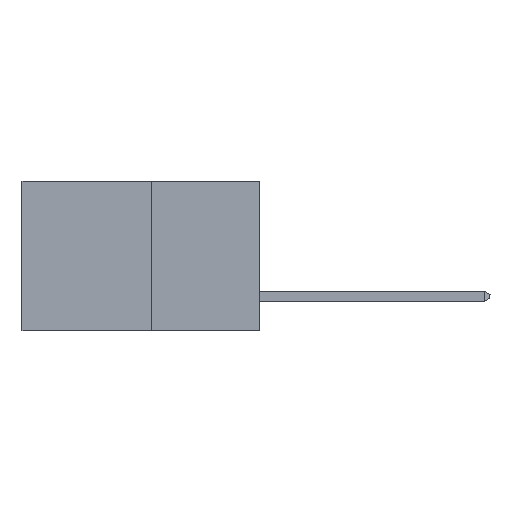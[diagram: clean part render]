
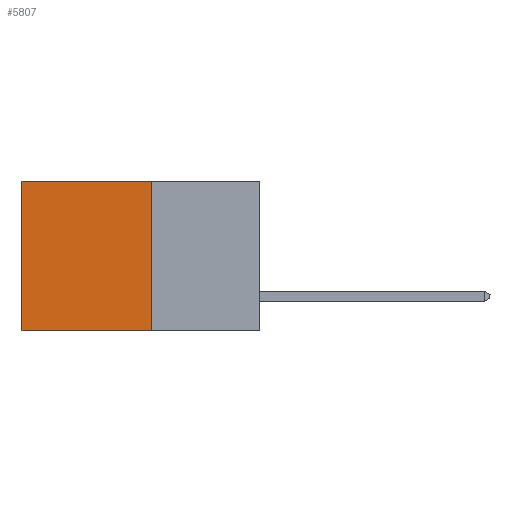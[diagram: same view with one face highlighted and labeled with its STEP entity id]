
A CAD part, left-side view. The second image highlights one B-rep face of the part: STEP entity #5807.
In plain terms, the highlighted planar face has unit normal (-1, 0, 0).
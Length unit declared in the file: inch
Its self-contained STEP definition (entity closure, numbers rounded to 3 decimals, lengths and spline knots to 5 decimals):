
#302 = EDGE_CURVE ( 'NONE', #2329, #4702, #9518, .T. ) ;
#835 = EDGE_CURVE ( 'NONE', #9638, #2329, #3325, .T. ) ;
#1392 = CARTESIAN_POINT ( 'NONE',  ( 0.277, 0.27, -0.37 ) ) ;
#1440 = CARTESIAN_POINT ( 'NONE',  ( 0.277, 0.59, -0.37 ) ) ;
#2182 = DIRECTION ( 'NONE',  ( 1., 0., 0. ) ) ;
#2254 = VECTOR ( 'NONE', #4793, 39.37008 ) ;
#2329 = VERTEX_POINT ( 'NONE', #8815 ) ;
#2535 = DIRECTION ( 'NONE',  ( 0., 1., 0. ) ) ;
#2850 = ORIENTED_EDGE ( 'NONE', *, *, #6032, .T. ) ;
#3080 = CARTESIAN_POINT ( 'NONE',  ( 0.277, 0.27, 0. ) ) ;
#3222 = CARTESIAN_POINT ( 'NONE',  ( 0.277, 0.27, -0.37 ) ) ;
#3325 = LINE ( 'NONE', #3765, #9315 ) ;
#3765 = CARTESIAN_POINT ( 'NONE',  ( 0.277, 0.27, -0.37 ) ) ;
#3973 = CARTESIAN_POINT ( 'NONE',  ( 0.277, 0.59, -0.37 ) ) ;
#4070 = ORIENTED_EDGE ( 'NONE', *, *, #302, .F. ) ;
#4257 = FACE_OUTER_BOUND ( 'NONE', #5937, .T. ) ;
#4597 = VECTOR ( 'NONE', #2535, 39.37008 ) ;
#4702 = VERTEX_POINT ( 'NONE', #1440 ) ;
#4793 = DIRECTION ( 'NONE',  ( 0., 0., -1. ) ) ;
#4994 = AXIS2_PLACEMENT_3D ( 'NONE', #1392, #2182, #7740 ) ;
#5807 = ADVANCED_FACE ( 'NONE', ( #4257 ), #6152, .F. ) ;
#5937 = EDGE_LOOP ( 'NONE', ( #2850, #4070, #7294, #8297 ) ) ;
#6032 = EDGE_CURVE ( 'NONE', #6517, #4702, #8548, .T. ) ;
#6152 = PLANE ( 'NONE',  #4994 ) ;
#6195 = CARTESIAN_POINT ( 'NONE',  ( 0.277, 0.59, 0. ) ) ;
#6517 = VERTEX_POINT ( 'NONE', #6195 ) ;
#6573 = DIRECTION ( 'NONE',  ( 0., 0., -1. ) ) ;
#7261 = VECTOR ( 'NONE', #9210, 39.37008 ) ;
#7294 = ORIENTED_EDGE ( 'NONE', *, *, #835, .F. ) ;
#7296 = CARTESIAN_POINT ( 'NONE',  ( 0.277, 0.27, 0. ) ) ;
#7740 = DIRECTION ( 'NONE',  ( 0., 0., -1. ) ) ;
#8297 = ORIENTED_EDGE ( 'NONE', *, *, #8699, .T. ) ;
#8509 = LINE ( 'NONE', #7296, #4597 ) ;
#8548 = LINE ( 'NONE', #3973, #2254 ) ;
#8699 = EDGE_CURVE ( 'NONE', #9638, #6517, #8509, .T. ) ;
#8815 = CARTESIAN_POINT ( 'NONE',  ( 0.277, 0.27, -0.37 ) ) ;
#9210 = DIRECTION ( 'NONE',  ( 0., 1., 0. ) ) ;
#9315 = VECTOR ( 'NONE', #6573, 39.37008 ) ;
#9518 = LINE ( 'NONE', #3222, #7261 ) ;
#9638 = VERTEX_POINT ( 'NONE', #3080 ) ;
